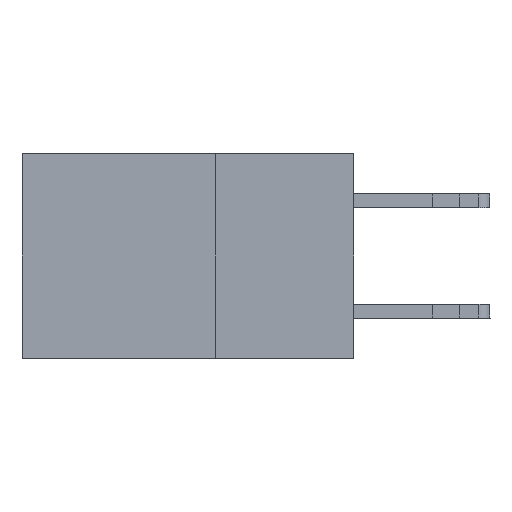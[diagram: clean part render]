
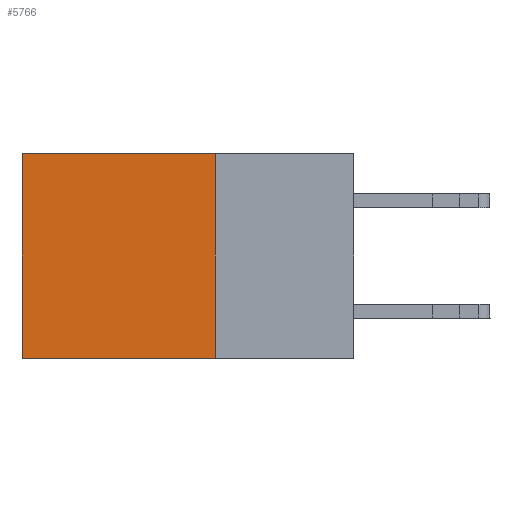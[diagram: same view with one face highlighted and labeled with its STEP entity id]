
A CAD part, left-side view. The second image highlights one B-rep face of the part: STEP entity #5766.
In plain terms, the highlighted planar face has unit normal (-1, 0, 0).
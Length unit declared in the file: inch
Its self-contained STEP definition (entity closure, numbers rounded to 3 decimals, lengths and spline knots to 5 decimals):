
#169 = VECTOR ( 'NONE', #1911, 39.37008 ) ;
#205 = VECTOR ( 'NONE', #4668, 39.37008 ) ;
#1428 = PLANE ( 'NONE',  #16843 ) ;
#1451 = CARTESIAN_POINT ( 'NONE',  ( 0.2875, 0.6, -0.37 ) ) ;
#1911 = DIRECTION ( 'NONE',  ( 0., 1., 0. ) ) ;
#2779 = VERTEX_POINT ( 'NONE', #1451 ) ;
#2926 = DIRECTION ( 'NONE',  ( 1., 0., 0. ) ) ;
#2973 = DIRECTION ( 'NONE',  ( 0., 0., -1. ) ) ;
#3320 = CARTESIAN_POINT ( 'NONE',  ( 0.2875, 0.6, 0. ) ) ;
#3382 = VECTOR ( 'NONE', #13280, 39.37008 ) ;
#4015 = CARTESIAN_POINT ( 'NONE',  ( 0.2875, 0.6, 0. ) ) ;
#4668 = DIRECTION ( 'NONE',  ( 0., 1., 0. ) ) ;
#5766 = ADVANCED_FACE ( 'NONE', ( #13503 ), #1428, .F. ) ;
#5857 = VECTOR ( 'NONE', #2973, 39.37008 ) ;
#6045 = CARTESIAN_POINT ( 'NONE',  ( 0.2875, 0.25, -0.37 ) ) ;
#7429 = LINE ( 'NONE', #4015, #3382 ) ;
#7500 = ORIENTED_EDGE ( 'NONE', *, *, #16031, .T. ) ;
#8323 = LINE ( 'NONE', #18584, #205 ) ;
#10459 = EDGE_CURVE ( 'NONE', #16085, #2779, #7429, .T. ) ;
#10625 = CARTESIAN_POINT ( 'NONE',  ( 0.2875, 0.25, 0. ) ) ;
#11151 = ORIENTED_EDGE ( 'NONE', *, *, #17697, .F. ) ;
#12144 = CARTESIAN_POINT ( 'NONE',  ( 0.2875, 0.25, 0. ) ) ;
#13280 = DIRECTION ( 'NONE',  ( 0., 0., -1. ) ) ;
#13503 = FACE_OUTER_BOUND ( 'NONE', #17696, .T. ) ;
#13725 = DIRECTION ( 'NONE',  ( 0., 0., -1. ) ) ;
#14409 = VERTEX_POINT ( 'NONE', #6045 ) ;
#15610 = CARTESIAN_POINT ( 'NONE',  ( 0.2875, 0.25, -0.37 ) ) ;
#16031 = EDGE_CURVE ( 'NONE', #16261, #16085, #8323, .T. ) ;
#16085 = VERTEX_POINT ( 'NONE', #3320 ) ;
#16261 = VERTEX_POINT ( 'NONE', #19043 ) ;
#16576 = EDGE_CURVE ( 'NONE', #16261, #14409, #18198, .T. ) ;
#16843 = AXIS2_PLACEMENT_3D ( 'NONE', #12144, #2926, #13725 ) ;
#16960 = LINE ( 'NONE', #15610, #169 ) ;
#17696 = EDGE_LOOP ( 'NONE', ( #18854, #11151, #19329, #7500 ) ) ;
#17697 = EDGE_CURVE ( 'NONE', #14409, #2779, #16960, .T. ) ;
#18198 = LINE ( 'NONE', #10625, #5857 ) ;
#18584 = CARTESIAN_POINT ( 'NONE',  ( 0.2875, 0.25, 0. ) ) ;
#18854 = ORIENTED_EDGE ( 'NONE', *, *, #10459, .T. ) ;
#19043 = CARTESIAN_POINT ( 'NONE',  ( 0.2875, 0.25, 0. ) ) ;
#19329 = ORIENTED_EDGE ( 'NONE', *, *, #16576, .F. ) ;
